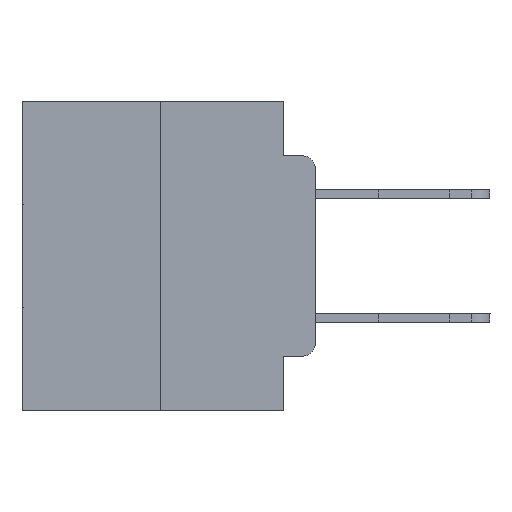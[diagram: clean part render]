
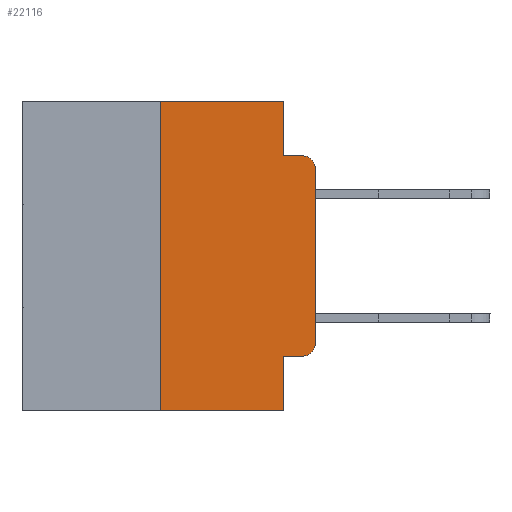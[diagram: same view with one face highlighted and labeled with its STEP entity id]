
A CAD part, left-side view. The second image highlights one B-rep face of the part: STEP entity #22116.
In plain terms, the highlighted planar face has unit normal (-1, 0, 0).
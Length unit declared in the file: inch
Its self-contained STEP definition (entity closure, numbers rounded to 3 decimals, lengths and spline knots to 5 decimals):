
#294 = DIRECTION ( 'NONE',  ( 0., 0., -1. ) ) ;
#352 = CARTESIAN_POINT ( 'NONE',  ( 0., 0.473, -0.5 ) ) ;
#2740 = EDGE_LOOP ( 'NONE', ( #21816, #6372, #14502, #12837, #9138, #24250, #10745, #18349, #24057, #12646 ) ) ;
#2763 = DIRECTION ( 'NONE',  ( 0., 0., -1. ) ) ;
#2906 = AXIS2_PLACEMENT_3D ( 'NONE', #17245, #11182, #2763 ) ;
#3370 = EDGE_CURVE ( 'NONE', #23065, #8913, #21240, .T. ) ;
#3444 = EDGE_CURVE ( 'NONE', #13237, #19009, #8405, .T. ) ;
#3576 = DIRECTION ( 'NONE',  ( 0., 0., -1. ) ) ;
#4035 = VERTEX_POINT ( 'NONE', #6349 ) ;
#4689 = LINE ( 'NONE', #11436, #26825 ) ;
#5278 = LINE ( 'NONE', #14420, #18119 ) ;
#5994 = EDGE_CURVE ( 'NONE', #11314, #13237, #4689, .T. ) ;
#6039 = DIRECTION ( 'NONE',  ( 0., -1., 0. ) ) ;
#6096 = CARTESIAN_POINT ( 'NONE',  ( 0., 0.02, -0.0885 ) ) ;
#6244 = VECTOR ( 'NONE', #294, 39.37008 ) ;
#6349 = CARTESIAN_POINT ( 'NONE',  ( 0., 0.25, -0.5 ) ) ;
#6372 = ORIENTED_EDGE ( 'NONE', *, *, #3444, .T. ) ;
#6711 = CARTESIAN_POINT ( 'NONE',  ( 0., 0., -0.3915 ) ) ;
#6995 = CARTESIAN_POINT ( 'NONE',  ( 0., 0.051, -0.5 ) ) ;
#7222 = CARTESIAN_POINT ( 'NONE',  ( 0., 0.051, -0.0885 ) ) ;
#7431 = VERTEX_POINT ( 'NONE', #6995 ) ;
#7645 = DIRECTION ( 'NONE',  ( 0., 0., -1. ) ) ;
#8405 = CIRCLE ( 'NONE', #24335, 0.02 ) ;
#8576 = LINE ( 'NONE', #21539, #6244 ) ;
#8617 = CIRCLE ( 'NONE', #17992, 0.02 ) ;
#8913 = VERTEX_POINT ( 'NONE', #7222 ) ;
#8915 = LINE ( 'NONE', #21259, #13826 ) ;
#9057 = DIRECTION ( 'NONE',  ( 0., 0., 1. ) ) ;
#9138 = ORIENTED_EDGE ( 'NONE', *, *, #13163, .F. ) ;
#9670 = LINE ( 'NONE', #352, #14288 ) ;
#10048 = DIRECTION ( 'NONE',  ( 0., -1., 0. ) ) ;
#10745 = ORIENTED_EDGE ( 'NONE', *, *, #12771, .T. ) ;
#11182 = DIRECTION ( 'NONE',  ( 1., 0., 0. ) ) ;
#11314 = VERTEX_POINT ( 'NONE', #6711 ) ;
#11360 = VERTEX_POINT ( 'NONE', #19441 ) ;
#11436 = CARTESIAN_POINT ( 'NONE',  ( 0., 0., 0. ) ) ;
#11541 = EDGE_CURVE ( 'NONE', #11360, #21594, #16653, .T. ) ;
#11690 = CARTESIAN_POINT ( 'NONE',  ( 0., 0.051, -0.4115 ) ) ;
#11868 = DIRECTION ( 'NONE',  ( -1., 0., 0. ) ) ;
#12222 = DIRECTION ( 'NONE',  ( 0., -1., 0. ) ) ;
#12646 = ORIENTED_EDGE ( 'NONE', *, *, #14383, .T. ) ;
#12741 = VERTEX_POINT ( 'NONE', #23245 ) ;
#12771 = EDGE_CURVE ( 'NONE', #4035, #7431, #9670, .T. ) ;
#12837 = ORIENTED_EDGE ( 'NONE', *, *, #3370, .F. ) ;
#12940 = LINE ( 'NONE', #22577, #17887 ) ;
#13163 = EDGE_CURVE ( 'NONE', #12741, #23065, #12940, .T. ) ;
#13237 = VERTEX_POINT ( 'NONE', #22667 ) ;
#13826 = VECTOR ( 'NONE', #21626, 39.37008 ) ;
#14288 = VECTOR ( 'NONE', #21407, 39.37008 ) ;
#14383 = EDGE_CURVE ( 'NONE', #21594, #11314, #8617, .T. ) ;
#14420 = CARTESIAN_POINT ( 'NONE',  ( 0., 0.051, -0.0885 ) ) ;
#14502 = ORIENTED_EDGE ( 'NONE', *, *, #23164, .F. ) ;
#15609 = VECTOR ( 'NONE', #15964, 39.37008 ) ;
#15964 = DIRECTION ( 'NONE',  ( 0., 0., -1. ) ) ;
#16653 = LINE ( 'NONE', #11690, #18652 ) ;
#17187 = FACE_OUTER_BOUND ( 'NONE', #2740, .T. ) ;
#17245 = CARTESIAN_POINT ( 'NONE',  ( 0., 0.473, 0. ) ) ;
#17515 = PLANE ( 'NONE',  #2906 ) ;
#17887 = VECTOR ( 'NONE', #10048, 39.37008 ) ;
#17992 = AXIS2_PLACEMENT_3D ( 'NONE', #26891, #11868, #7645 ) ;
#18119 = VECTOR ( 'NONE', #6039, 39.37008 ) ;
#18349 = ORIENTED_EDGE ( 'NONE', *, *, #23349, .F. ) ;
#18652 = VECTOR ( 'NONE', #12222, 39.37008 ) ;
#19009 = VERTEX_POINT ( 'NONE', #6096 ) ;
#19441 = CARTESIAN_POINT ( 'NONE',  ( 0., 0.051, -0.4115 ) ) ;
#20451 = CARTESIAN_POINT ( 'NONE',  ( 0., 0.051, 0. ) ) ;
#20694 = DIRECTION ( 'NONE',  ( -1., 0., 0. ) ) ;
#21240 = LINE ( 'NONE', #22078, #15609 ) ;
#21259 = CARTESIAN_POINT ( 'NONE',  ( 0., 0.25, 0. ) ) ;
#21407 = DIRECTION ( 'NONE',  ( 0., -1., 0. ) ) ;
#21539 = CARTESIAN_POINT ( 'NONE',  ( 0., 0.051, 0. ) ) ;
#21594 = VERTEX_POINT ( 'NONE', #22660 ) ;
#21626 = DIRECTION ( 'NONE',  ( 0., 0., 1. ) ) ;
#21816 = ORIENTED_EDGE ( 'NONE', *, *, #5994, .T. ) ;
#22078 = CARTESIAN_POINT ( 'NONE',  ( 0., 0.051, 0. ) ) ;
#22116 = ADVANCED_FACE ( 'NONE', ( #17187 ), #17515, .F. ) ;
#22577 = CARTESIAN_POINT ( 'NONE',  ( 0., 0.473, 0. ) ) ;
#22660 = CARTESIAN_POINT ( 'NONE',  ( 0., 0.02, -0.4115 ) ) ;
#22667 = CARTESIAN_POINT ( 'NONE',  ( 0., 0., -0.1085 ) ) ;
#23065 = VERTEX_POINT ( 'NONE', #20451 ) ;
#23164 = EDGE_CURVE ( 'NONE', #8913, #19009, #5278, .T. ) ;
#23245 = CARTESIAN_POINT ( 'NONE',  ( 0., 0.25, 0. ) ) ;
#23349 = EDGE_CURVE ( 'NONE', #11360, #7431, #8576, .T. ) ;
#23354 = EDGE_CURVE ( 'NONE', #4035, #12741, #8915, .T. ) ;
#24057 = ORIENTED_EDGE ( 'NONE', *, *, #11541, .T. ) ;
#24250 = ORIENTED_EDGE ( 'NONE', *, *, #23354, .F. ) ;
#24335 = AXIS2_PLACEMENT_3D ( 'NONE', #26768, #20694, #3576 ) ;
#26768 = CARTESIAN_POINT ( 'NONE',  ( 0., 0.02, -0.1085 ) ) ;
#26825 = VECTOR ( 'NONE', #9057, 39.37008 ) ;
#26891 = CARTESIAN_POINT ( 'NONE',  ( 0., 0.02, -0.3915 ) ) ;
